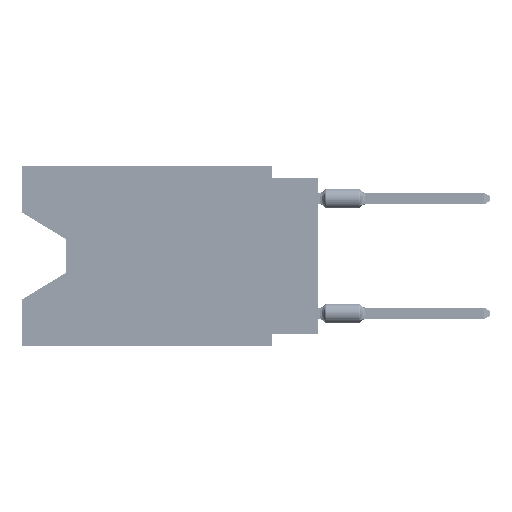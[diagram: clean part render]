
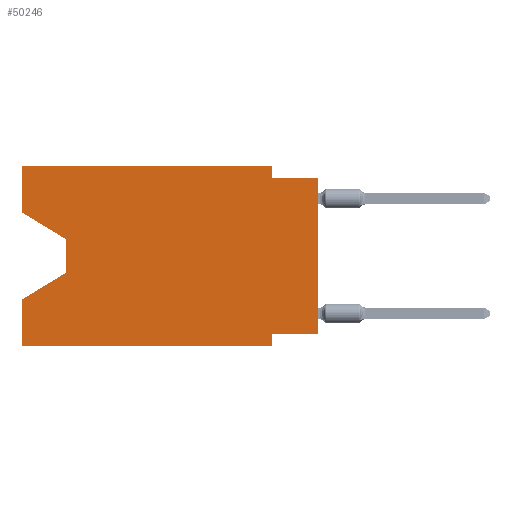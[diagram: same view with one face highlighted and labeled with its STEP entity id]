
A CAD part, left-side view. The second image highlights one B-rep face of the part: STEP entity #50246.
In plain terms, the highlighted planar face has unit normal (-1, 0, 0).
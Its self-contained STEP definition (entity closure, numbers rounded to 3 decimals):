
#35 = VECTOR ( 'NONE', #1976, 1000. ) ;
#232 = CARTESIAN_POINT ( 'NONE',  ( 0., 2.54, 0. ) ) ;
#981 = CARTESIAN_POINT ( 'NONE',  ( 0., 2.54, -9.906 ) ) ;
#1521 = VECTOR ( 'NONE', #28576, 1000. ) ;
#1760 = CARTESIAN_POINT ( 'NONE',  ( 0., 0., -9.271 ) ) ;
#1976 = DIRECTION ( 'NONE',  ( 0., 0.855, -0.519 ) ) ;
#2045 = LINE ( 'NONE', #31139, #69548 ) ;
#2081 = LINE ( 'NONE', #981, #40519 ) ;
#2778 = VECTOR ( 'NONE', #26546, 1000. ) ;
#2887 = EDGE_CURVE ( 'NONE', #66529, #14182, #2045, .T. ) ;
#4604 = VECTOR ( 'NONE', #47266, 1000. ) ;
#4875 = DIRECTION ( 'NONE',  ( 0., -1., 0. ) ) ;
#5364 = ORIENTED_EDGE ( 'NONE', *, *, #73250, .F. ) ;
#5752 = EDGE_LOOP ( 'NONE', ( #30752, #56157, #31859, #58848, #12660, #5364, #55499, #16054, #34430, #51647, #56555, #64706 ) ) ;
#8270 = DIRECTION ( 'NONE',  ( 0., 0., -1. ) ) ;
#9127 = VECTOR ( 'NONE', #19860, 1000. ) ;
#9605 = EDGE_CURVE ( 'NONE', #51349, #23128, #38718, .T. ) ;
#10276 = CARTESIAN_POINT ( 'NONE',  ( 0., 16.383, 0. ) ) ;
#10355 = VECTOR ( 'NONE', #13438, 1000. ) ;
#11271 = DIRECTION ( 'NONE',  ( 0., 0., -1. ) ) ;
#11636 = PLANE ( 'NONE',  #33116 ) ;
#12169 = DIRECTION ( 'NONE',  ( 0., 0., 1. ) ) ;
#12660 = ORIENTED_EDGE ( 'NONE', *, *, #2887, .T. ) ;
#13438 = DIRECTION ( 'NONE',  ( 0., 0., 1. ) ) ;
#14182 = VERTEX_POINT ( 'NONE', #61715 ) ;
#16054 = ORIENTED_EDGE ( 'NONE', *, *, #19975, .T. ) ;
#17668 = VERTEX_POINT ( 'NONE', #50057 ) ;
#18399 = EDGE_CURVE ( 'NONE', #39822, #17668, #47630, .T. ) ;
#19860 = DIRECTION ( 'NONE',  ( 0., -0.855, -0.519 ) ) ;
#19975 = EDGE_CURVE ( 'NONE', #63882, #17668, #35207, .T. ) ;
#20905 = EDGE_CURVE ( 'NONE', #63882, #38901, #35396, .T. ) ;
#21664 = CARTESIAN_POINT ( 'NONE',  ( 0., 2.54, -0.635 ) ) ;
#23128 = VERTEX_POINT ( 'NONE', #42641 ) ;
#26491 = CARTESIAN_POINT ( 'NONE',  ( 0., 16.383, 0. ) ) ;
#26546 = DIRECTION ( 'NONE',  ( 0., 0., 1. ) ) ;
#27394 = CARTESIAN_POINT ( 'NONE',  ( 0., 16.383, -2.546 ) ) ;
#28514 = EDGE_CURVE ( 'NONE', #57841, #36562, #31067, .T. ) ;
#28576 = DIRECTION ( 'NONE',  ( 0., 0., -1. ) ) ;
#29081 = CARTESIAN_POINT ( 'NONE',  ( 0., 16.383, -7.36 ) ) ;
#30198 = LINE ( 'NONE', #70607, #70177 ) ;
#30752 = ORIENTED_EDGE ( 'NONE', *, *, #9605, .T. ) ;
#30840 = DIRECTION ( 'NONE',  ( 0., 1., 0. ) ) ;
#31067 = LINE ( 'NONE', #47693, #35 ) ;
#31139 = CARTESIAN_POINT ( 'NONE',  ( 0., 16.383, -9.906 ) ) ;
#31859 = ORIENTED_EDGE ( 'NONE', *, *, #28514, .T. ) ;
#33116 = AXIS2_PLACEMENT_3D ( 'NONE', #70163, #58800, #11271 ) ;
#33236 = EDGE_CURVE ( 'NONE', #51836, #39822, #57258, .T. ) ;
#34430 = ORIENTED_EDGE ( 'NONE', *, *, #18399, .F. ) ;
#34887 = CARTESIAN_POINT ( 'NONE',  ( 0., 16.383, -9.906 ) ) ;
#35195 = CARTESIAN_POINT ( 'NONE',  ( 0., 0., -0.635 ) ) ;
#35207 = LINE ( 'NONE', #74499, #74130 ) ;
#35396 = LINE ( 'NONE', #1760, #57348 ) ;
#35916 = CARTESIAN_POINT ( 'NONE',  ( 0., 13.97, -5.893 ) ) ;
#36562 = VERTEX_POINT ( 'NONE', #29081 ) ;
#38718 = LINE ( 'NONE', #27394, #9127 ) ;
#38901 = VERTEX_POINT ( 'NONE', #61319 ) ;
#39822 = VERTEX_POINT ( 'NONE', #21664 ) ;
#40299 = CARTESIAN_POINT ( 'NONE',  ( 0., 2.54, 0. ) ) ;
#40358 = LINE ( 'NONE', #56610, #51201 ) ;
#40519 = VECTOR ( 'NONE', #58741, 1000. ) ;
#42157 = CARTESIAN_POINT ( 'NONE',  ( 0., 16.383, 0. ) ) ;
#42469 = CARTESIAN_POINT ( 'NONE',  ( 0., 0., -9.271 ) ) ;
#42641 = CARTESIAN_POINT ( 'NONE',  ( 0., 13.97, -4.013 ) ) ;
#47266 = DIRECTION ( 'NONE',  ( 0., -1., 0. ) ) ;
#47393 = DIRECTION ( 'NONE',  ( 0., -1., 0. ) ) ;
#47630 = LINE ( 'NONE', #35195, #4604 ) ;
#47693 = CARTESIAN_POINT ( 'NONE',  ( 0., 13.97, -5.893 ) ) ;
#50057 = CARTESIAN_POINT ( 'NONE',  ( 0., 0., -0.635 ) ) ;
#50246 = ADVANCED_FACE ( 'NONE', ( #57333 ), #11636, .F. ) ;
#51201 = VECTOR ( 'NONE', #4875, 1000. ) ;
#51349 = VERTEX_POINT ( 'NONE', #55587 ) ;
#51647 = ORIENTED_EDGE ( 'NONE', *, *, #33236, .F. ) ;
#51836 = VERTEX_POINT ( 'NONE', #40299 ) ;
#52051 = EDGE_CURVE ( 'NONE', #51349, #54186, #71229, .T. ) ;
#54186 = VERTEX_POINT ( 'NONE', #26491 ) ;
#55499 = ORIENTED_EDGE ( 'NONE', *, *, #20905, .F. ) ;
#55587 = CARTESIAN_POINT ( 'NONE',  ( 0., 16.383, -2.546 ) ) ;
#56157 = ORIENTED_EDGE ( 'NONE', *, *, #61388, .T. ) ;
#56555 = ORIENTED_EDGE ( 'NONE', *, *, #71507, .F. ) ;
#56610 = CARTESIAN_POINT ( 'NONE',  ( 0., 16.383, 0. ) ) ;
#57258 = LINE ( 'NONE', #232, #1521 ) ;
#57333 = FACE_OUTER_BOUND ( 'NONE', #5752, .T. ) ;
#57348 = VECTOR ( 'NONE', #30840, 1000. ) ;
#57841 = VERTEX_POINT ( 'NONE', #35916 ) ;
#58741 = DIRECTION ( 'NONE',  ( 0., 0., -1. ) ) ;
#58800 = DIRECTION ( 'NONE',  ( 1., 0., 0. ) ) ;
#58848 = ORIENTED_EDGE ( 'NONE', *, *, #69973, .F. ) ;
#61319 = CARTESIAN_POINT ( 'NONE',  ( 0., 2.54, -9.271 ) ) ;
#61388 = EDGE_CURVE ( 'NONE', #23128, #57841, #30198, .T. ) ;
#61715 = CARTESIAN_POINT ( 'NONE',  ( 0., 2.54, -9.906 ) ) ;
#63882 = VERTEX_POINT ( 'NONE', #42469 ) ;
#64706 = ORIENTED_EDGE ( 'NONE', *, *, #52051, .F. ) ;
#66529 = VERTEX_POINT ( 'NONE', #34887 ) ;
#69548 = VECTOR ( 'NONE', #47393, 1000. ) ;
#69973 = EDGE_CURVE ( 'NONE', #66529, #36562, #72976, .T. ) ;
#70163 = CARTESIAN_POINT ( 'NONE',  ( 0., 16.383, 0. ) ) ;
#70177 = VECTOR ( 'NONE', #8270, 1000. ) ;
#70607 = CARTESIAN_POINT ( 'NONE',  ( 0., 13.97, -4.013 ) ) ;
#71229 = LINE ( 'NONE', #42157, #10355 ) ;
#71507 = EDGE_CURVE ( 'NONE', #54186, #51836, #40358, .T. ) ;
#72976 = LINE ( 'NONE', #10276, #2778 ) ;
#73250 = EDGE_CURVE ( 'NONE', #38901, #14182, #2081, .T. ) ;
#74130 = VECTOR ( 'NONE', #12169, 1000. ) ;
#74499 = CARTESIAN_POINT ( 'NONE',  ( 0., 0., 0. ) ) ;
